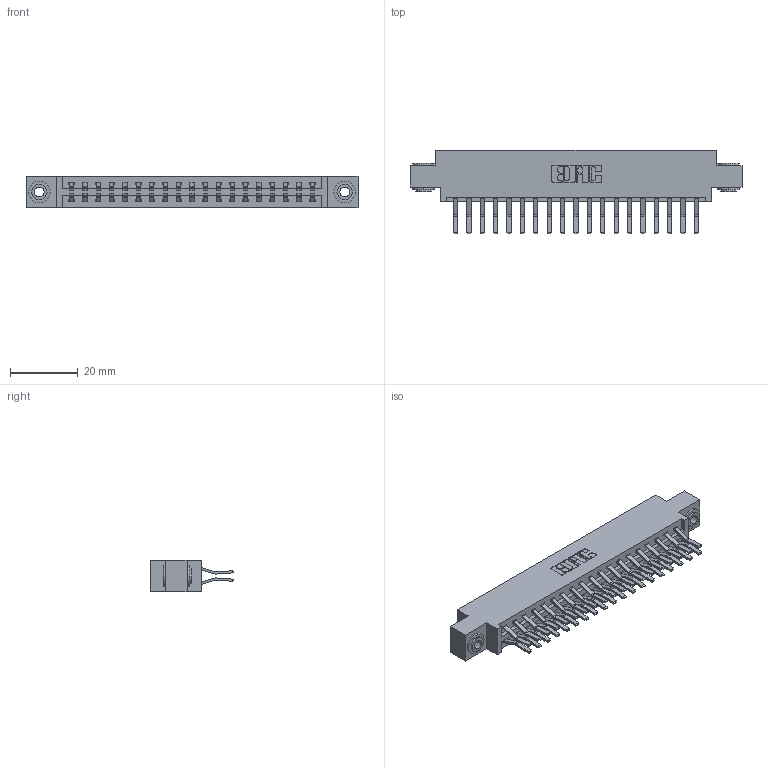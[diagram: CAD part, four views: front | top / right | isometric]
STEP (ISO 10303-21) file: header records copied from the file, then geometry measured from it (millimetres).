
FILE_DESCRIPTION (( 'STEP AP203' ), '1' );
FILE_NAME ('337-038-560-803.STEP', '2018-08-08T06:22:16', ( '' ), ( '' ), 'SwSTEP 2.0', 'SolidWorks 2016', '' );
FILE_SCHEMA (( 'CONFIG_CONTROL_DESIGN' ));
Length unit declared in the file: inch
Products named in the file (4): 337-038-560-803; 337 Part_0.170 Offset - 0.156 Dia-TH; 345-292-001_560 Tail; 345-250-002_345-250-002-102
Assembly tree (41 placements, depth 2):
  337-038-560-803
    337 Part_0.170 Offset - 0.156 Dia-TH
    345-292-001_560 Tail  x38
    345-250-002_345-250-002-102  x2
Bounding box: 98.3 x 24.78 x 9.4 mm (x, y, z)
Volume: 10204.2 mm3; surface area: 12365.6 mm2
Topology: 41 solids, 41 shells, 2284 faces, 6745 edges, 4442 vertices
Faces by surface type: plane 1528, cylinder 748, cone 8
Entity records: 18576 total; most frequent: CARTESIAN_POINT 3125, ORIENTED_EDGE 3054, DIRECTION 2737, EDGE_CURVE 1527, VECTOR 1371, LINE 1371, VERTEX_POINT 1014, AXIS2_PLACEMENT_3D 683
